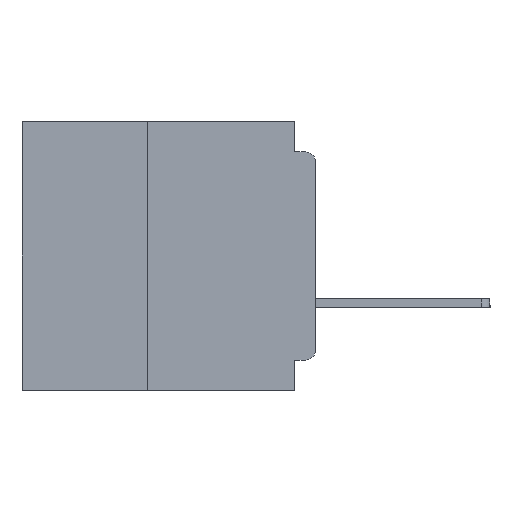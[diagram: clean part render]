
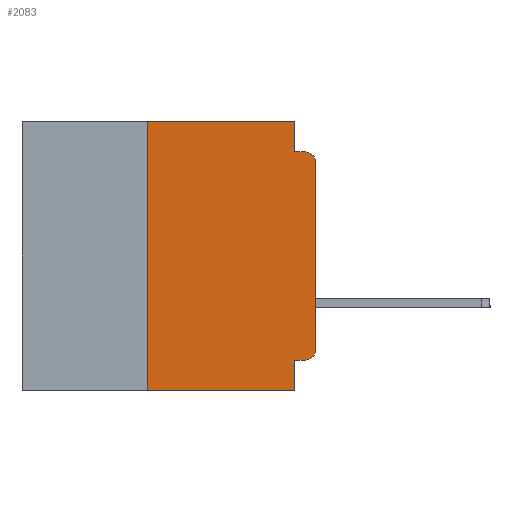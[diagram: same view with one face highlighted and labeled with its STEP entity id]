
A CAD part, left-side view. The second image highlights one B-rep face of the part: STEP entity #2083.
In plain terms, the highlighted planar face has unit normal (-1, 0, 0).
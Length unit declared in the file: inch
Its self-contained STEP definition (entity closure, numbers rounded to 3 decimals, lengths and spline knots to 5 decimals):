
#143 = EDGE_CURVE ( 'NONE', #24122, #28632, #271, .T. ) ;
#271 = CIRCLE ( 'NONE', #7820, 0.015 ) ;
#374 = EDGE_CURVE ( 'NONE', #5214, #6962, #30779, .T. ) ;
#429 = LINE ( 'NONE', #11381, #19301 ) ;
#586 = EDGE_CURVE ( 'NONE', #6822, #20950, #11568, .T. ) ;
#664 = CARTESIAN_POINT ( 'NONE',  ( 0., 0., -0.355 ) ) ;
#1676 = LINE ( 'NONE', #5520, #2868 ) ;
#2083 = ADVANCED_FACE ( 'NONE', ( #20648 ), #45253, .F. ) ;
#2868 = VECTOR ( 'NONE', #27845, 39.37008 ) ;
#2908 = EDGE_CURVE ( 'NONE', #33878, #20950, #32806, .T. ) ;
#3399 = ORIENTED_EDGE ( 'NONE', *, *, #586, .T. ) ;
#4107 = VERTEX_POINT ( 'NONE', #5513 ) ;
#4833 = LINE ( 'NONE', #40159, #43428 ) ;
#4943 = ORIENTED_EDGE ( 'NONE', *, *, #2908, .F. ) ;
#4979 = EDGE_CURVE ( 'NONE', #28632, #5214, #6371, .T. ) ;
#5214 = VERTEX_POINT ( 'NONE', #38652 ) ;
#5312 = ORIENTED_EDGE ( 'NONE', *, *, #6036, .F. ) ;
#5324 = VERTEX_POINT ( 'NONE', #5692 ) ;
#5513 = CARTESIAN_POINT ( 'NONE',  ( 0., 0.031, -0.045 ) ) ;
#5520 = CARTESIAN_POINT ( 'NONE',  ( 0., 0.25, -0.4 ) ) ;
#5692 = CARTESIAN_POINT ( 'NONE',  ( 0., 0.031, 0. ) ) ;
#6036 = EDGE_CURVE ( 'NONE', #4107, #6962, #26196, .T. ) ;
#6371 = LINE ( 'NONE', #37218, #24960 ) ;
#6634 = ORIENTED_EDGE ( 'NONE', *, *, #23441, .F. ) ;
#6822 = VERTEX_POINT ( 'NONE', #14302 ) ;
#6962 = VERTEX_POINT ( 'NONE', #26745 ) ;
#7082 = ORIENTED_EDGE ( 'NONE', *, *, #4979, .T. ) ;
#7567 = CARTESIAN_POINT ( 'NONE',  ( 0., 0.015, -0.355 ) ) ;
#7632 = DIRECTION ( 'NONE',  ( 0., -1., 0. ) ) ;
#7820 = AXIS2_PLACEMENT_3D ( 'NONE', #45715, #45601, #45554 ) ;
#8840 = AXIS2_PLACEMENT_3D ( 'NONE', #45309, #44924, #44704 ) ;
#8936 = LINE ( 'NONE', #664, #47369 ) ;
#9944 = DIRECTION ( 'NONE',  ( 0., -1., 0. ) ) ;
#11195 = DIRECTION ( 'NONE',  ( 0., 0., 1. ) ) ;
#11381 = CARTESIAN_POINT ( 'NONE',  ( 0., 0.437, 0. ) ) ;
#11568 = LINE ( 'NONE', #26756, #40091 ) ;
#14302 = CARTESIAN_POINT ( 'NONE',  ( 0., 0.25, -0.4 ) ) ;
#16394 = VECTOR ( 'NONE', #9944, 39.37008 ) ;
#18894 = VERTEX_POINT ( 'NONE', #20164 ) ;
#19301 = VECTOR ( 'NONE', #7632, 39.37008 ) ;
#20164 = CARTESIAN_POINT ( 'NONE',  ( 0., 0.25, 0. ) ) ;
#20648 = FACE_OUTER_BOUND ( 'NONE', #38893, .T. ) ;
#20950 = VERTEX_POINT ( 'NONE', #33325 ) ;
#23441 = EDGE_CURVE ( 'NONE', #6822, #18894, #1676, .T. ) ;
#24122 = VERTEX_POINT ( 'NONE', #7567 ) ;
#24272 = AXIS2_PLACEMENT_3D ( 'NONE', #34055, #33997, #33941 ) ;
#24960 = VECTOR ( 'NONE', #11195, 39.37008 ) ;
#26196 = LINE ( 'NONE', #43364, #16394 ) ;
#26745 = CARTESIAN_POINT ( 'NONE',  ( 0., 0.015, -0.045 ) ) ;
#26756 = CARTESIAN_POINT ( 'NONE',  ( 0., 0.437, -0.4 ) ) ;
#26967 = DIRECTION ( 'NONE',  ( 0., -1., 0. ) ) ;
#27845 = DIRECTION ( 'NONE',  ( 0., 0., 1. ) ) ;
#28632 = VERTEX_POINT ( 'NONE', #42790 ) ;
#30779 = CIRCLE ( 'NONE', #24272, 0.015 ) ;
#32517 = EDGE_CURVE ( 'NONE', #5324, #4107, #4833, .T. ) ;
#32626 = DIRECTION ( 'NONE',  ( 0., 0., -1. ) ) ;
#32806 = LINE ( 'NONE', #42506, #42799 ) ;
#33325 = CARTESIAN_POINT ( 'NONE',  ( 0., 0.031, -0.4 ) ) ;
#33460 = EDGE_CURVE ( 'NONE', #24122, #33878, #8936, .T. ) ;
#33804 = ORIENTED_EDGE ( 'NONE', *, *, #143, .T. ) ;
#33878 = VERTEX_POINT ( 'NONE', #40907 ) ;
#33941 = DIRECTION ( 'NONE',  ( 0., 0., -1. ) ) ;
#33997 = DIRECTION ( 'NONE',  ( -1., 0., 0. ) ) ;
#34055 = CARTESIAN_POINT ( 'NONE',  ( 0., 0.015, -0.06 ) ) ;
#35983 = ORIENTED_EDGE ( 'NONE', *, *, #36235, .F. ) ;
#36235 = EDGE_CURVE ( 'NONE', #18894, #5324, #429, .T. ) ;
#37218 = CARTESIAN_POINT ( 'NONE',  ( 0., 0., 0. ) ) ;
#38168 = DIRECTION ( 'NONE',  ( 0., 1., 0. ) ) ;
#38470 = ORIENTED_EDGE ( 'NONE', *, *, #374, .T. ) ;
#38652 = CARTESIAN_POINT ( 'NONE',  ( 0., 0., -0.06 ) ) ;
#38893 = EDGE_LOOP ( 'NONE', ( #7082, #38470, #5312, #45096, #35983, #6634, #3399, #4943, #40899, #33804 ) ) ;
#40091 = VECTOR ( 'NONE', #26967, 39.37008 ) ;
#40159 = CARTESIAN_POINT ( 'NONE',  ( 0., 0.031, 0. ) ) ;
#40899 = ORIENTED_EDGE ( 'NONE', *, *, #33460, .F. ) ;
#40907 = CARTESIAN_POINT ( 'NONE',  ( 0., 0.031, -0.355 ) ) ;
#41751 = DIRECTION ( 'NONE',  ( 0., 0., -1. ) ) ;
#42506 = CARTESIAN_POINT ( 'NONE',  ( 0., 0.031, -0.4 ) ) ;
#42790 = CARTESIAN_POINT ( 'NONE',  ( 0., 0., -0.34 ) ) ;
#42799 = VECTOR ( 'NONE', #41751, 39.37008 ) ;
#43364 = CARTESIAN_POINT ( 'NONE',  ( 0., 0., -0.045 ) ) ;
#43428 = VECTOR ( 'NONE', #32626, 39.37008 ) ;
#44704 = DIRECTION ( 'NONE',  ( 0., 0., -1. ) ) ;
#44924 = DIRECTION ( 'NONE',  ( 1., 0., 0. ) ) ;
#45096 = ORIENTED_EDGE ( 'NONE', *, *, #32517, .F. ) ;
#45253 = PLANE ( 'NONE',  #8840 ) ;
#45309 = CARTESIAN_POINT ( 'NONE',  ( 0., 0.437, 0. ) ) ;
#45554 = DIRECTION ( 'NONE',  ( 0., 0., -1. ) ) ;
#45601 = DIRECTION ( 'NONE',  ( -1., 0., 0. ) ) ;
#45715 = CARTESIAN_POINT ( 'NONE',  ( 0., 0.015, -0.34 ) ) ;
#47369 = VECTOR ( 'NONE', #38168, 39.37008 ) ;
